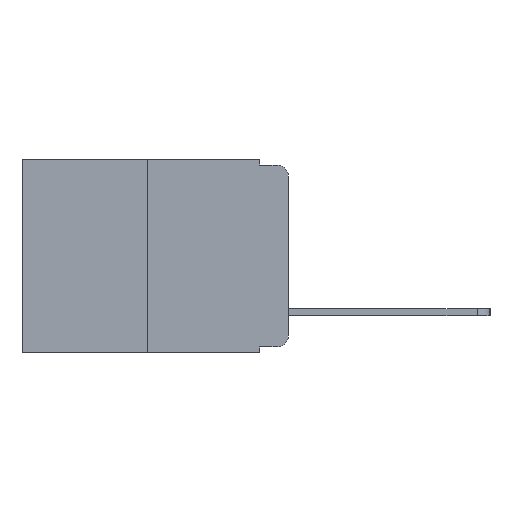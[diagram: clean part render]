
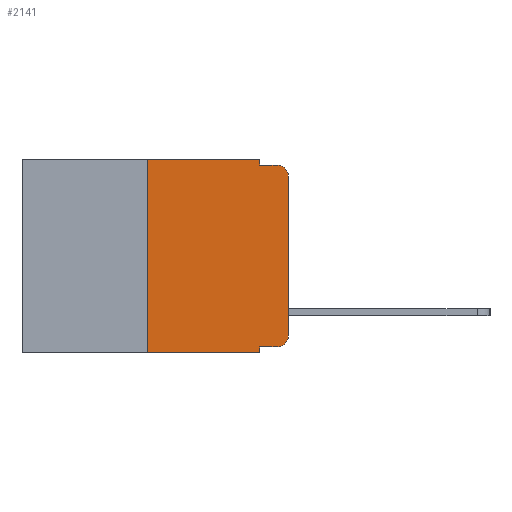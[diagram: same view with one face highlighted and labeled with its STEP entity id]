
A CAD part, left-side view. The second image highlights one B-rep face of the part: STEP entity #2141.
In plain terms, the highlighted planar face has unit normal (-1, 0, 0).
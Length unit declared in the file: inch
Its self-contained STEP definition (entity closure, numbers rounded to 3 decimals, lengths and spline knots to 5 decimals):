
#53 = VECTOR ( 'NONE', #12050, 39.37008 ) ;
#240 = VERTEX_POINT ( 'NONE', #10374 ) ;
#560 = VERTEX_POINT ( 'NONE', #4680 ) ;
#705 = CARTESIAN_POINT ( 'NONE',  ( 0., 0.473, -0.343 ) ) ;
#1332 = DIRECTION ( 'NONE',  ( 0., 0., -1. ) ) ;
#1723 = CARTESIAN_POINT ( 'NONE',  ( 0., 0.473, 0. ) ) ;
#1773 = DIRECTION ( 'NONE',  ( 1., 0., 0. ) ) ;
#2075 = DIRECTION ( 'NONE',  ( 0., 0., -1. ) ) ;
#2141 = ADVANCED_FACE ( 'NONE', ( #6802 ), #5522, .F. ) ;
#2510 = CARTESIAN_POINT ( 'NONE',  ( 0., 0., -0.313 ) ) ;
#2521 = DIRECTION ( 'NONE',  ( 0., 0., -1. ) ) ;
#2576 = CARTESIAN_POINT ( 'NONE',  ( 0., 0.25, -0.343 ) ) ;
#2878 = CARTESIAN_POINT ( 'NONE',  ( 0., 0.051, -0.01 ) ) ;
#2935 = VECTOR ( 'NONE', #1332, 39.37008 ) ;
#2938 = DIRECTION ( 'NONE',  ( 0., -1., 0. ) ) ;
#3082 = CARTESIAN_POINT ( 'NONE',  ( 0., 0.02, -0.01 ) ) ;
#3434 = EDGE_CURVE ( 'NONE', #11883, #6556, #5548, .T. ) ;
#3675 = AXIS2_PLACEMENT_3D ( 'NONE', #14252, #6218, #2521 ) ;
#3900 = DIRECTION ( 'NONE',  ( 0., 0., 1. ) ) ;
#3964 = LINE ( 'NONE', #1723, #9650 ) ;
#4680 = CARTESIAN_POINT ( 'NONE',  ( 0., 0., -0.03 ) ) ;
#4770 = DIRECTION ( 'NONE',  ( 0., 0., -1. ) ) ;
#5084 = AXIS2_PLACEMENT_3D ( 'NONE', #5529, #1773, #2075 ) ;
#5257 = EDGE_CURVE ( 'NONE', #560, #11174, #8508, .T. ) ;
#5522 = PLANE ( 'NONE',  #5084 ) ;
#5529 = CARTESIAN_POINT ( 'NONE',  ( 0., 0.473, 0. ) ) ;
#5548 = CIRCLE ( 'NONE', #14001, 0.02 ) ;
#5718 = VECTOR ( 'NONE', #2938, 39.37008 ) ;
#5979 = LINE ( 'NONE', #8227, #2935 ) ;
#6218 = DIRECTION ( 'NONE',  ( -1., 0., 0. ) ) ;
#6329 = DIRECTION ( 'NONE',  ( 0., -1., 0. ) ) ;
#6382 = CARTESIAN_POINT ( 'NONE',  ( 0., 0.051, -0.333 ) ) ;
#6556 = VERTEX_POINT ( 'NONE', #2510 ) ;
#6589 = LINE ( 'NONE', #705, #53 ) ;
#6716 = DIRECTION ( 'NONE',  ( -1., 0., 0. ) ) ;
#6749 = EDGE_CURVE ( 'NONE', #240, #11174, #13353, .T. ) ;
#6802 = FACE_OUTER_BOUND ( 'NONE', #12630, .T. ) ;
#6917 = DIRECTION ( 'NONE',  ( 0., 0., -1. ) ) ;
#7303 = VERTEX_POINT ( 'NONE', #13827 ) ;
#7851 = VERTEX_POINT ( 'NONE', #2576 ) ;
#8056 = CARTESIAN_POINT ( 'NONE',  ( 0., 0.051, -0.343 ) ) ;
#8063 = LINE ( 'NONE', #8463, #13480 ) ;
#8227 = CARTESIAN_POINT ( 'NONE',  ( 0., 0.051, 0. ) ) ;
#8288 = EDGE_CURVE ( 'NONE', #10863, #240, #5979, .T. ) ;
#8426 = CARTESIAN_POINT ( 'NONE',  ( 0., 0., 0. ) ) ;
#8447 = ORIENTED_EDGE ( 'NONE', *, *, #9246, .T. ) ;
#8463 = CARTESIAN_POINT ( 'NONE',  ( 0., 0.25, 0. ) ) ;
#8508 = CIRCLE ( 'NONE', #3675, 0.02 ) ;
#8615 = DIRECTION ( 'NONE',  ( 0., -1., 0. ) ) ;
#8729 = CARTESIAN_POINT ( 'NONE',  ( 0., 0.25, 0. ) ) ;
#9163 = ORIENTED_EDGE ( 'NONE', *, *, #6749, .F. ) ;
#9180 = ORIENTED_EDGE ( 'NONE', *, *, #5257, .T. ) ;
#9246 = EDGE_CURVE ( 'NONE', #6556, #560, #10548, .T. ) ;
#9317 = ORIENTED_EDGE ( 'NONE', *, *, #8288, .F. ) ;
#9596 = DIRECTION ( 'NONE',  ( 0., 0., 1. ) ) ;
#9650 = VECTOR ( 'NONE', #8615, 39.37008 ) ;
#9748 = ORIENTED_EDGE ( 'NONE', *, *, #9810, .F. ) ;
#9760 = LINE ( 'NONE', #14538, #12254 ) ;
#9810 = EDGE_CURVE ( 'NONE', #7851, #11365, #8063, .T. ) ;
#9858 = VECTOR ( 'NONE', #3900, 39.37008 ) ;
#9885 = ORIENTED_EDGE ( 'NONE', *, *, #9905, .F. ) ;
#9905 = EDGE_CURVE ( 'NONE', #11365, #10863, #3964, .T. ) ;
#9931 = ORIENTED_EDGE ( 'NONE', *, *, #10608, .T. ) ;
#10199 = ORIENTED_EDGE ( 'NONE', *, *, #12658, .F. ) ;
#10224 = VERTEX_POINT ( 'NONE', #8056 ) ;
#10274 = ORIENTED_EDGE ( 'NONE', *, *, #14061, .T. ) ;
#10374 = CARTESIAN_POINT ( 'NONE',  ( 0., 0.051, -0.01 ) ) ;
#10548 = LINE ( 'NONE', #8426, #9858 ) ;
#10608 = EDGE_CURVE ( 'NONE', #7851, #10224, #6589, .T. ) ;
#10863 = VERTEX_POINT ( 'NONE', #12502 ) ;
#11174 = VERTEX_POINT ( 'NONE', #3082 ) ;
#11316 = LINE ( 'NONE', #6382, #5718 ) ;
#11365 = VERTEX_POINT ( 'NONE', #8729 ) ;
#11883 = VERTEX_POINT ( 'NONE', #14102 ) ;
#12050 = DIRECTION ( 'NONE',  ( 0., -1., 0. ) ) ;
#12254 = VECTOR ( 'NONE', #6917, 39.37008 ) ;
#12502 = CARTESIAN_POINT ( 'NONE',  ( 0., 0.051, 0. ) ) ;
#12630 = EDGE_LOOP ( 'NONE', ( #8447, #9180, #9163, #9317, #9885, #9748, #9931, #10199, #10274, #12663 ) ) ;
#12658 = EDGE_CURVE ( 'NONE', #7303, #10224, #9760, .T. ) ;
#12663 = ORIENTED_EDGE ( 'NONE', *, *, #3434, .T. ) ;
#13013 = VECTOR ( 'NONE', #6329, 39.37008 ) ;
#13353 = LINE ( 'NONE', #2878, #13013 ) ;
#13437 = CARTESIAN_POINT ( 'NONE',  ( 0., 0.02, -0.313 ) ) ;
#13480 = VECTOR ( 'NONE', #9596, 39.37008 ) ;
#13827 = CARTESIAN_POINT ( 'NONE',  ( 0., 0.051, -0.333 ) ) ;
#14001 = AXIS2_PLACEMENT_3D ( 'NONE', #13437, #6716, #4770 ) ;
#14061 = EDGE_CURVE ( 'NONE', #7303, #11883, #11316, .T. ) ;
#14102 = CARTESIAN_POINT ( 'NONE',  ( 0., 0.02, -0.333 ) ) ;
#14252 = CARTESIAN_POINT ( 'NONE',  ( 0., 0.02, -0.03 ) ) ;
#14538 = CARTESIAN_POINT ( 'NONE',  ( 0., 0.051, 0. ) ) ;
